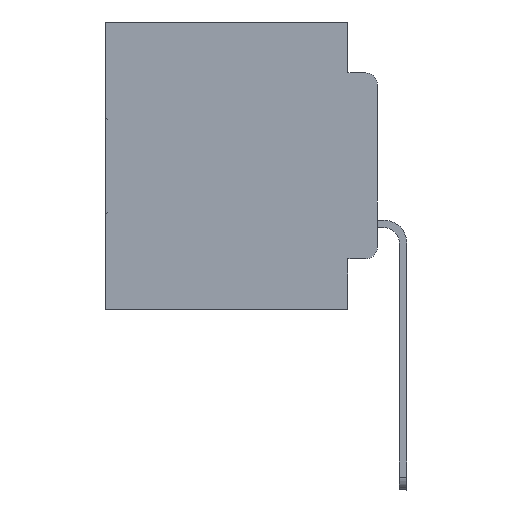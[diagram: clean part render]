
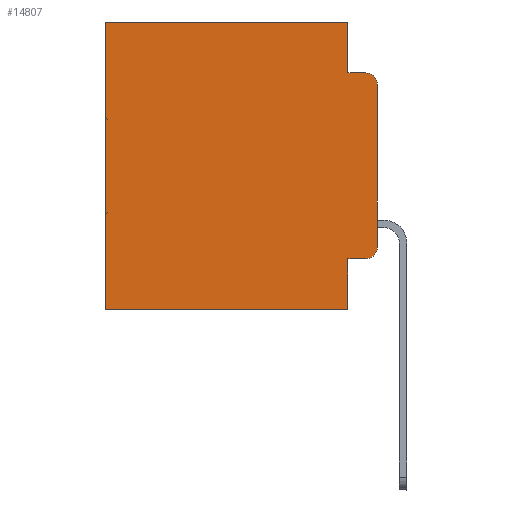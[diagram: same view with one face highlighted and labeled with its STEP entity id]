
A CAD part, left-side view. The second image highlights one B-rep face of the part: STEP entity #14807.
In plain terms, the highlighted planar face has unit normal (-1, 0, 0).
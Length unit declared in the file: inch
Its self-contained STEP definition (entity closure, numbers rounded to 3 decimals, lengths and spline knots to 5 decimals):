
#29 = CARTESIAN_POINT ( 'NONE',  ( 0.298, 0., -0.1085 ) ) ;
#576 = FACE_OUTER_BOUND ( 'NONE', #2331, .T. ) ;
#751 = DIRECTION ( 'NONE',  ( 0., 1., 0. ) ) ;
#859 = ORIENTED_EDGE ( 'NONE', *, *, #5751, .T. ) ;
#899 = DIRECTION ( 'NONE',  ( 0., -1., 0. ) ) ;
#1485 = CARTESIAN_POINT ( 'NONE',  ( 0.298, 0.051, -0.5 ) ) ;
#2331 = EDGE_LOOP ( 'NONE', ( #32048, #23706, #26271, #15487, #28310, #6599, #7630, #3937, #26906, #859 ) ) ;
#3183 = PLANE ( 'NONE',  #21565 ) ;
#3611 = VECTOR ( 'NONE', #28728, 39.37008 ) ;
#3640 = CARTESIAN_POINT ( 'NONE',  ( 0.298, 0., 0. ) ) ;
#3937 = ORIENTED_EDGE ( 'NONE', *, *, #26434, .F. ) ;
#4454 = CARTESIAN_POINT ( 'NONE',  ( 0.298, 0.02, -0.4115 ) ) ;
#5712 = VECTOR ( 'NONE', #899, 39.37008 ) ;
#5751 = EDGE_CURVE ( 'NONE', #6610, #12947, #29451, .T. ) ;
#5777 = CARTESIAN_POINT ( 'NONE',  ( 0.298, 0.051, -0.0885 ) ) ;
#5885 = LINE ( 'NONE', #20197, #11399 ) ;
#6418 = LINE ( 'NONE', #17898, #14342 ) ;
#6599 = ORIENTED_EDGE ( 'NONE', *, *, #15782, .T. ) ;
#6610 = VERTEX_POINT ( 'NONE', #4454 ) ;
#7248 = LINE ( 'NONE', #30264, #15160 ) ;
#7630 = ORIENTED_EDGE ( 'NONE', *, *, #26843, .F. ) ;
#8494 = CARTESIAN_POINT ( 'NONE',  ( 0.298, 0., -0.5 ) ) ;
#8499 = EDGE_CURVE ( 'NONE', #26497, #6610, #5885, .T. ) ;
#8602 = CARTESIAN_POINT ( 'NONE',  ( 0.298, 0.473, 0. ) ) ;
#8945 = DIRECTION ( 'NONE',  ( -1., 0., 0. ) ) ;
#9082 = AXIS2_PLACEMENT_3D ( 'NONE', #22714, #30147, #17468 ) ;
#9086 = VECTOR ( 'NONE', #32170, 39.37008 ) ;
#9285 = CARTESIAN_POINT ( 'NONE',  ( 0.298, 0.051, 0. ) ) ;
#10438 = DIRECTION ( 'NONE',  ( 0., 1., 0. ) ) ;
#10775 = VERTEX_POINT ( 'NONE', #24760 ) ;
#11399 = VECTOR ( 'NONE', #25760, 39.37008 ) ;
#12902 = CARTESIAN_POINT ( 'NONE',  ( 0.298, 0., 0. ) ) ;
#12941 = DIRECTION ( 'NONE',  ( 0., 0., -1. ) ) ;
#12947 = VERTEX_POINT ( 'NONE', #26547 ) ;
#13167 = CARTESIAN_POINT ( 'NONE',  ( 0.298, 0.051, 0. ) ) ;
#13576 = EDGE_CURVE ( 'NONE', #23124, #10775, #21286, .T. ) ;
#13595 = CARTESIAN_POINT ( 'NONE',  ( 0.298, 0.051, -0.0885 ) ) ;
#14342 = VECTOR ( 'NONE', #10438, 39.37008 ) ;
#14807 = ADVANCED_FACE ( 'NONE', ( #576 ), #3183, .F. ) ;
#15160 = VECTOR ( 'NONE', #27509, 39.37008 ) ;
#15394 = EDGE_CURVE ( 'NONE', #32738, #10775, #25556, .T. ) ;
#15464 = DIRECTION ( 'NONE',  ( 0., 0., -1. ) ) ;
#15487 = ORIENTED_EDGE ( 'NONE', *, *, #26758, .F. ) ;
#15782 = EDGE_CURVE ( 'NONE', #16070, #27122, #7248, .T. ) ;
#16070 = VERTEX_POINT ( 'NONE', #8602 ) ;
#16226 = LINE ( 'NONE', #8494, #29733 ) ;
#16564 = EDGE_CURVE ( 'NONE', #31446, #16070, #6418, .T. ) ;
#17468 = DIRECTION ( 'NONE',  ( 0., 0., -1. ) ) ;
#17898 = CARTESIAN_POINT ( 'NONE',  ( 0.298, 0., 0. ) ) ;
#18007 = DIRECTION ( 'NONE',  ( 1., 0., 0. ) ) ;
#19890 = EDGE_CURVE ( 'NONE', #23124, #12947, #31811, .T. ) ;
#20099 = VERTEX_POINT ( 'NONE', #1485 ) ;
#20197 = CARTESIAN_POINT ( 'NONE',  ( 0.298, 0.051, -0.4115 ) ) ;
#21286 = CIRCLE ( 'NONE', #29610, 0.02 ) ;
#21565 = AXIS2_PLACEMENT_3D ( 'NONE', #12902, #18007, #15464 ) ;
#22714 = CARTESIAN_POINT ( 'NONE',  ( 0.298, 0.02, -0.3915 ) ) ;
#23124 = VERTEX_POINT ( 'NONE', #29 ) ;
#23706 = ORIENTED_EDGE ( 'NONE', *, *, #13576, .T. ) ;
#24289 = CARTESIAN_POINT ( 'NONE',  ( 0.298, 0.02, -0.1085 ) ) ;
#24760 = CARTESIAN_POINT ( 'NONE',  ( 0.298, 0.02, -0.0885 ) ) ;
#24806 = CARTESIAN_POINT ( 'NONE',  ( 0.298, 0.473, -0.5 ) ) ;
#25556 = LINE ( 'NONE', #5777, #5712 ) ;
#25760 = DIRECTION ( 'NONE',  ( 0., -1., 0. ) ) ;
#26271 = ORIENTED_EDGE ( 'NONE', *, *, #15394, .F. ) ;
#26434 = EDGE_CURVE ( 'NONE', #26497, #20099, #28597, .T. ) ;
#26497 = VERTEX_POINT ( 'NONE', #32375 ) ;
#26547 = CARTESIAN_POINT ( 'NONE',  ( 0.298, 0., -0.3915 ) ) ;
#26615 = LINE ( 'NONE', #13167, #30148 ) ;
#26758 = EDGE_CURVE ( 'NONE', #31446, #32738, #26615, .T. ) ;
#26816 = CARTESIAN_POINT ( 'NONE',  ( 0.298, 0.051, 0. ) ) ;
#26843 = EDGE_CURVE ( 'NONE', #20099, #27122, #16226, .T. ) ;
#26906 = ORIENTED_EDGE ( 'NONE', *, *, #8499, .T. ) ;
#27122 = VERTEX_POINT ( 'NONE', #24806 ) ;
#27509 = DIRECTION ( 'NONE',  ( 0., 0., -1. ) ) ;
#28310 = ORIENTED_EDGE ( 'NONE', *, *, #16564, .T. ) ;
#28597 = LINE ( 'NONE', #9285, #9086 ) ;
#28728 = DIRECTION ( 'NONE',  ( 0., 0., -1. ) ) ;
#28964 = DIRECTION ( 'NONE',  ( 0., 0., -1. ) ) ;
#29451 = CIRCLE ( 'NONE', #9082, 0.02 ) ;
#29610 = AXIS2_PLACEMENT_3D ( 'NONE', #24289, #8945, #28964 ) ;
#29733 = VECTOR ( 'NONE', #751, 39.37008 ) ;
#30147 = DIRECTION ( 'NONE',  ( -1., 0., 0. ) ) ;
#30148 = VECTOR ( 'NONE', #12941, 39.37008 ) ;
#30264 = CARTESIAN_POINT ( 'NONE',  ( 0.298, 0.473, 0. ) ) ;
#31446 = VERTEX_POINT ( 'NONE', #26816 ) ;
#31811 = LINE ( 'NONE', #3640, #3611 ) ;
#32048 = ORIENTED_EDGE ( 'NONE', *, *, #19890, .F. ) ;
#32170 = DIRECTION ( 'NONE',  ( 0., 0., -1. ) ) ;
#32375 = CARTESIAN_POINT ( 'NONE',  ( 0.298, 0.051, -0.4115 ) ) ;
#32738 = VERTEX_POINT ( 'NONE', #13595 ) ;
